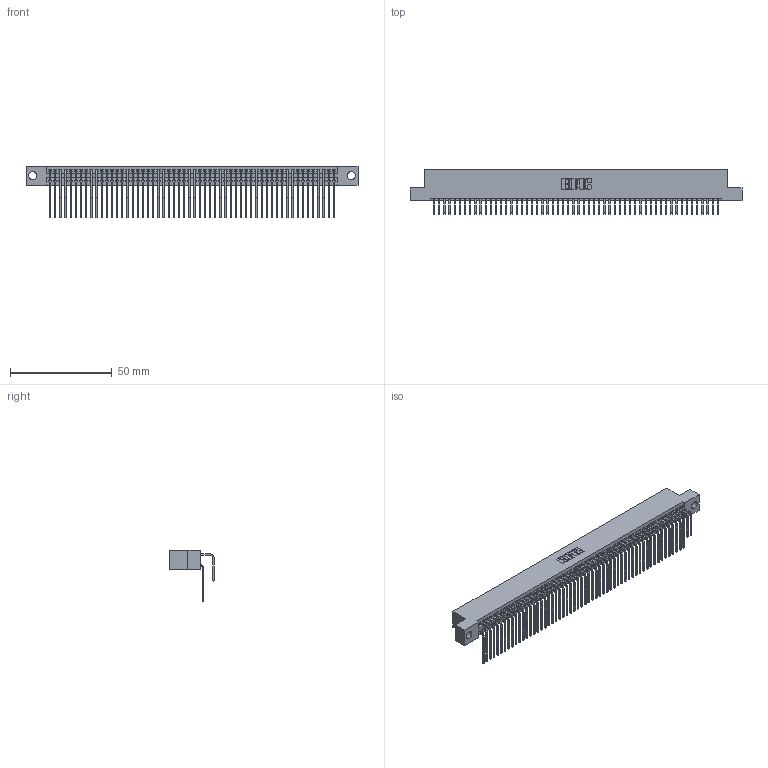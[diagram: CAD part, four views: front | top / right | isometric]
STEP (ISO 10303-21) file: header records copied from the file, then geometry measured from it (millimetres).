
FILE_DESCRIPTION (( 'STEP AP203' ), '1' );
FILE_NAME ('345-112-558-204.STEP', '2021-05-25T14:41:35', ( '' ), ( '' ), 'SwSTEP 2.0', 'SolidWorks 2020', '' );
FILE_SCHEMA (( 'CONFIG_CONTROL_DESIGN' ));
Length unit declared in the file: inch
Products named in the file (4): 345 Part_Flush Mounting Lugs - 0.156 Dia-TI; 345-292-001_558 Tail - 2; 345-112-558-204; 345-292-001_558 559 Tail - 1
Assembly tree (113 placements, depth 2):
  345-112-558-204
    345 Part_Flush Mounting Lugs - 0.156 Dia-TI
    345-292-001_558 559 Tail - 1  x56
    345-292-001_558 Tail - 2  x56
Bounding box: 163.45 x 21.83 x 25.53 mm (x, y, z)
Volume: 16547.7 mm3; surface area: 27621.2 mm2
Topology: 113 solids, 113 shells, 5964 faces, 17737 edges, 11674 vertices
Faces by surface type: plane 4014, cylinder 1950
Entity records: 44125 total; most frequent: CARTESIAN_POINT 7433, ORIENTED_EDGE 7314, DIRECTION 6509, EDGE_CURVE 3657, LINE 3261, VECTOR 3261, VERTEX_POINT 2434, AXIS2_PLACEMENT_3D 1624
